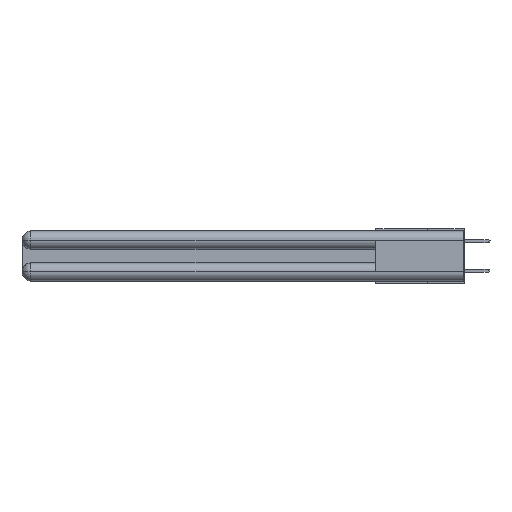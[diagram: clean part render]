
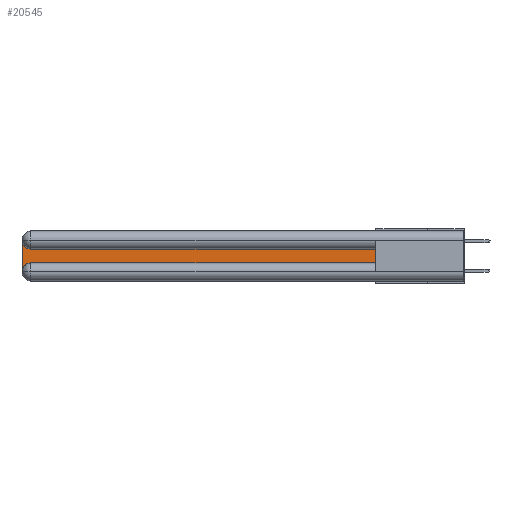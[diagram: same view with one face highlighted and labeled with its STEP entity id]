
A CAD part, left-side view. The second image highlights one B-rep face of the part: STEP entity #20545.
In plain terms, the highlighted planar face has unit normal (-1, 0, 0).
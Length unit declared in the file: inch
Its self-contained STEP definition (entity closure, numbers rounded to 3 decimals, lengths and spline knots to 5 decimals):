
#830 = VERTEX_POINT ( 'NONE', #11386 ) ;
#1635 = CARTESIAN_POINT ( 'NONE',  ( 0.075, 0.6, -0.2175 ) ) ;
#1740 = VERTEX_POINT ( 'NONE', #22572 ) ;
#2336 = AXIS2_PLACEMENT_3D ( 'NONE', #6956, #22920, #25182 ) ;
#2368 = VECTOR ( 'NONE', #8363, 39.37008 ) ;
#4572 = VECTOR ( 'NONE', #10073, 39.37008 ) ;
#5053 = CARTESIAN_POINT ( 'NONE',  ( 0.075, 2.94, -0.1225 ) ) ;
#5130 = LINE ( 'NONE', #25082, #16222 ) ;
#6058 = CARTESIAN_POINT ( 'NONE',  ( 0.075, 3., -0.1225 ) ) ;
#6090 = AXIS2_PLACEMENT_3D ( 'NONE', #27179, #20035, #13529 ) ;
#6788 = VERTEX_POINT ( 'NONE', #12584 ) ;
#6956 = CARTESIAN_POINT ( 'NONE',  ( 0.075, 2.94, -0.0625 ) ) ;
#7270 = AXIS2_PLACEMENT_3D ( 'NONE', #6058, #19535, #15009 ) ;
#7979 = CARTESIAN_POINT ( 'NONE',  ( 0.075, 0.6, -0.2175 ) ) ;
#8363 = DIRECTION ( 'NONE',  ( 0., 1., 0. ) ) ;
#8765 = EDGE_CURVE ( 'NONE', #21811, #830, #28673, .T. ) ;
#8776 = EDGE_CURVE ( 'NONE', #17099, #6788, #5130, .T. ) ;
#8791 = ORIENTED_EDGE ( 'NONE', *, *, #8776, .T. ) ;
#10073 = DIRECTION ( 'NONE',  ( 0., -1., 0. ) ) ;
#10274 = CARTESIAN_POINT ( 'NONE',  ( 0.075, 3., -0.2175 ) ) ;
#11386 = CARTESIAN_POINT ( 'NONE',  ( 0.075, 3., -0.0625 ) ) ;
#12584 = CARTESIAN_POINT ( 'NONE',  ( 0.075, 0.6, -0.1225 ) ) ;
#13529 = DIRECTION ( 'NONE',  ( 0., 0., -1. ) ) ;
#14134 = ORIENTED_EDGE ( 'NONE', *, *, #16179, .T. ) ;
#14975 = ORIENTED_EDGE ( 'NONE', *, *, #17477, .T. ) ;
#15009 = DIRECTION ( 'NONE',  ( 0., 0., -1. ) ) ;
#15143 = CARTESIAN_POINT ( 'NONE',  ( 0.075, 0.6, -0.1225 ) ) ;
#16179 = EDGE_CURVE ( 'NONE', #830, #1740, #25648, .T. ) ;
#16222 = VECTOR ( 'NONE', #23203, 39.37008 ) ;
#17099 = VERTEX_POINT ( 'NONE', #1635 ) ;
#17477 = EDGE_CURVE ( 'NONE', #1740, #28899, #23892, .T. ) ;
#19342 = EDGE_CURVE ( 'NONE', #28899, #17099, #26302, .T. ) ;
#19535 = DIRECTION ( 'NONE',  ( 1., 0., 0. ) ) ;
#20035 = DIRECTION ( 'NONE',  ( 1., 0., 0. ) ) ;
#20545 = ADVANCED_FACE ( 'NONE', ( #27321 ), #28469, .F. ) ;
#21382 = VECTOR ( 'NONE', #26210, 39.37008 ) ;
#21406 = EDGE_CURVE ( 'NONE', #6788, #21811, #28693, .T. ) ;
#21811 = VERTEX_POINT ( 'NONE', #5053 ) ;
#22572 = CARTESIAN_POINT ( 'NONE',  ( 0.075, 3., -0.2775 ) ) ;
#22584 = ORIENTED_EDGE ( 'NONE', *, *, #21406, .T. ) ;
#22748 = CARTESIAN_POINT ( 'NONE',  ( 0.075, 2.94, -0.2175 ) ) ;
#22920 = DIRECTION ( 'NONE',  ( 1., 0., 0. ) ) ;
#23203 = DIRECTION ( 'NONE',  ( 0., 0., 1. ) ) ;
#23892 = CIRCLE ( 'NONE', #6090, 0.06 ) ;
#24778 = ORIENTED_EDGE ( 'NONE', *, *, #19342, .T. ) ;
#25082 = CARTESIAN_POINT ( 'NONE',  ( 0.075, 0.6, -0.2175 ) ) ;
#25182 = DIRECTION ( 'NONE',  ( 0., 0., -1. ) ) ;
#25648 = LINE ( 'NONE', #10274, #21382 ) ;
#26005 = ORIENTED_EDGE ( 'NONE', *, *, #8765, .T. ) ;
#26210 = DIRECTION ( 'NONE',  ( 0., 0., -1. ) ) ;
#26302 = LINE ( 'NONE', #7979, #4572 ) ;
#27179 = CARTESIAN_POINT ( 'NONE',  ( 0.075, 2.94, -0.2775 ) ) ;
#27321 = FACE_OUTER_BOUND ( 'NONE', #29035, .T. ) ;
#28469 = PLANE ( 'NONE',  #7270 ) ;
#28673 = CIRCLE ( 'NONE', #2336, 0.06 ) ;
#28693 = LINE ( 'NONE', #15143, #2368 ) ;
#28899 = VERTEX_POINT ( 'NONE', #22748 ) ;
#29035 = EDGE_LOOP ( 'NONE', ( #22584, #26005, #14134, #14975, #24778, #8791 ) ) ;
